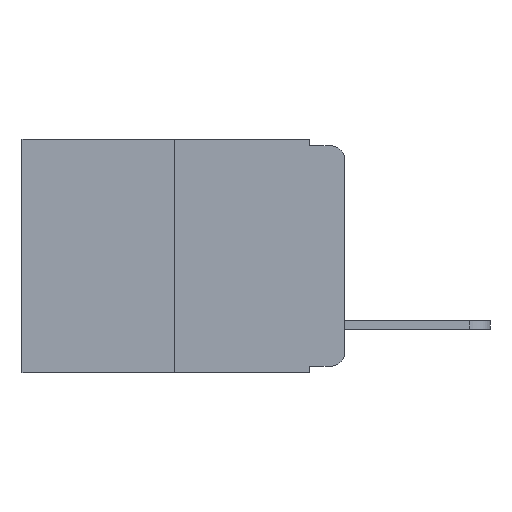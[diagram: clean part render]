
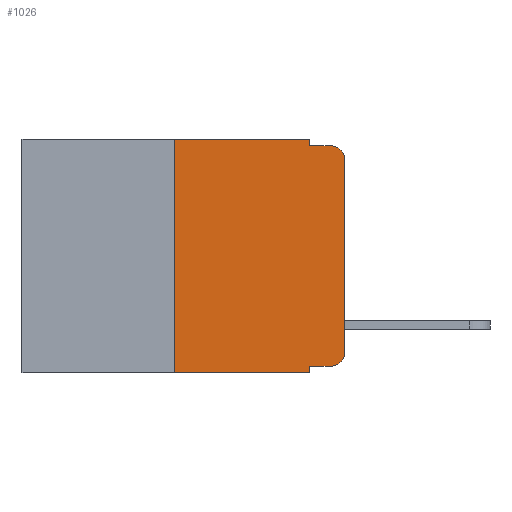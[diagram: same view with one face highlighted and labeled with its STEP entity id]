
A CAD part, left-side view. The second image highlights one B-rep face of the part: STEP entity #1026.
In plain terms, the highlighted planar face has unit normal (-1, 0, 0).
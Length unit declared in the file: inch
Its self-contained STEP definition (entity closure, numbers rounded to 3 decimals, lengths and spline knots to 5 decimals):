
#361 = AXIS2_PLACEMENT_3D ( 'NONE', #1355, #6761, #18345 ) ;
#426 = LINE ( 'NONE', #5913, #13586 ) ;
#1025 = ORIENTED_EDGE ( 'NONE', *, *, #10600, .T. ) ;
#1026 = ADVANCED_FACE ( 'NONE', ( #16637 ), #10312, .F. ) ;
#1355 = CARTESIAN_POINT ( 'NONE',  ( 0., 0.02, -0.03 ) ) ;
#1369 = CARTESIAN_POINT ( 'NONE',  ( 0., 0., 0. ) ) ;
#2298 = VECTOR ( 'NONE', #7303, 39.37008 ) ;
#2314 = CARTESIAN_POINT ( 'NONE',  ( 0., 0.051, 0. ) ) ;
#2365 = VERTEX_POINT ( 'NONE', #13059 ) ;
#3012 = ORIENTED_EDGE ( 'NONE', *, *, #4837, .T. ) ;
#3035 = LINE ( 'NONE', #8787, #15305 ) ;
#4790 = DIRECTION ( 'NONE',  ( 0., 0., -1. ) ) ;
#4837 = EDGE_CURVE ( 'NONE', #14351, #13334, #17825, .T. ) ;
#5016 = EDGE_CURVE ( 'NONE', #2365, #6572, #15844, .T. ) ;
#5109 = EDGE_LOOP ( 'NONE', ( #12586, #6023, #8458, #9532, #16990, #7857, #3012, #16229, #6933, #1025 ) ) ;
#5203 = VECTOR ( 'NONE', #17591, 39.37008 ) ;
#5406 = VERTEX_POINT ( 'NONE', #16628 ) ;
#5456 = CARTESIAN_POINT ( 'NONE',  ( 0., 0.02, -0.333 ) ) ;
#5725 = EDGE_CURVE ( 'NONE', #9122, #7414, #3035, .T. ) ;
#5913 = CARTESIAN_POINT ( 'NONE',  ( 0., 0.473, 0. ) ) ;
#6023 = ORIENTED_EDGE ( 'NONE', *, *, #6155, .T. ) ;
#6078 = DIRECTION ( 'NONE',  ( 1., 0., 0. ) ) ;
#6149 = DIRECTION ( 'NONE',  ( 0., -1., 0. ) ) ;
#6155 = EDGE_CURVE ( 'NONE', #5406, #13989, #14632, .T. ) ;
#6528 = CARTESIAN_POINT ( 'NONE',  ( 0., 0.473, -0.343 ) ) ;
#6572 = VERTEX_POINT ( 'NONE', #5456 ) ;
#6761 = DIRECTION ( 'NONE',  ( -1., 0., 0. ) ) ;
#6933 = ORIENTED_EDGE ( 'NONE', *, *, #5016, .T. ) ;
#7303 = DIRECTION ( 'NONE',  ( 0., 0., 1. ) ) ;
#7414 = VERTEX_POINT ( 'NONE', #11661 ) ;
#7448 = EDGE_CURVE ( 'NONE', #14351, #18371, #14358, .T. ) ;
#7857 = ORIENTED_EDGE ( 'NONE', *, *, #7448, .F. ) ;
#8193 = DIRECTION ( 'NONE',  ( 0., -1., 0. ) ) ;
#8458 = ORIENTED_EDGE ( 'NONE', *, *, #14794, .F. ) ;
#8787 = CARTESIAN_POINT ( 'NONE',  ( 0., 0.051, 0. ) ) ;
#9121 = AXIS2_PLACEMENT_3D ( 'NONE', #17445, #13130, #4790 ) ;
#9122 = VERTEX_POINT ( 'NONE', #2314 ) ;
#9532 = ORIENTED_EDGE ( 'NONE', *, *, #5725, .F. ) ;
#9575 = VECTOR ( 'NONE', #9656, 39.37008 ) ;
#9656 = DIRECTION ( 'NONE',  ( 0., -1., 0. ) ) ;
#9717 = CARTESIAN_POINT ( 'NONE',  ( 0., 0.25, -0.343 ) ) ;
#9768 = DIRECTION ( 'NONE',  ( 0., 0., 1. ) ) ;
#9975 = CARTESIAN_POINT ( 'NONE',  ( 0., 0.25, 0. ) ) ;
#10084 = CARTESIAN_POINT ( 'NONE',  ( 0., 0.25, 0. ) ) ;
#10249 = DIRECTION ( 'NONE',  ( 0., 0., -1. ) ) ;
#10312 = PLANE ( 'NONE',  #12602 ) ;
#10548 = CARTESIAN_POINT ( 'NONE',  ( 0., 0.051, -0.01 ) ) ;
#10600 = EDGE_CURVE ( 'NONE', #6572, #13340, #13796, .T. ) ;
#11089 = CARTESIAN_POINT ( 'NONE',  ( 0., 0.051, -0.333 ) ) ;
#11458 = EDGE_CURVE ( 'NONE', #13340, #5406, #17312, .T. ) ;
#11661 = CARTESIAN_POINT ( 'NONE',  ( 0., 0.051, -0.01 ) ) ;
#11980 = VECTOR ( 'NONE', #9768, 39.37008 ) ;
#12153 = CARTESIAN_POINT ( 'NONE',  ( 0., 0.051, -0.343 ) ) ;
#12586 = ORIENTED_EDGE ( 'NONE', *, *, #11458, .T. ) ;
#12602 = AXIS2_PLACEMENT_3D ( 'NONE', #15947, #6078, #16129 ) ;
#13059 = CARTESIAN_POINT ( 'NONE',  ( 0., 0.051, -0.333 ) ) ;
#13130 = DIRECTION ( 'NONE',  ( -1., 0., 0. ) ) ;
#13334 = VERTEX_POINT ( 'NONE', #12153 ) ;
#13340 = VERTEX_POINT ( 'NONE', #15016 ) ;
#13586 = VECTOR ( 'NONE', #6149, 39.37008 ) ;
#13707 = LINE ( 'NONE', #16288, #5203 ) ;
#13796 = CIRCLE ( 'NONE', #9121, 0.02 ) ;
#13989 = VERTEX_POINT ( 'NONE', #15924 ) ;
#14351 = VERTEX_POINT ( 'NONE', #9717 ) ;
#14358 = LINE ( 'NONE', #10084, #2298 ) ;
#14604 = EDGE_CURVE ( 'NONE', #18371, #9122, #426, .T. ) ;
#14632 = CIRCLE ( 'NONE', #361, 0.02 ) ;
#14794 = EDGE_CURVE ( 'NONE', #7414, #13989, #15841, .T. ) ;
#14828 = DIRECTION ( 'NONE',  ( 0., -1., 0. ) ) ;
#14930 = VECTOR ( 'NONE', #14828, 39.37008 ) ;
#15016 = CARTESIAN_POINT ( 'NONE',  ( 0., 0., -0.313 ) ) ;
#15305 = VECTOR ( 'NONE', #10249, 39.37008 ) ;
#15626 = VECTOR ( 'NONE', #8193, 39.37008 ) ;
#15841 = LINE ( 'NONE', #10548, #14930 ) ;
#15844 = LINE ( 'NONE', #11089, #9575 ) ;
#15924 = CARTESIAN_POINT ( 'NONE',  ( 0., 0.02, -0.01 ) ) ;
#15947 = CARTESIAN_POINT ( 'NONE',  ( 0., 0.473, 0. ) ) ;
#16129 = DIRECTION ( 'NONE',  ( 0., 0., -1. ) ) ;
#16229 = ORIENTED_EDGE ( 'NONE', *, *, #18019, .F. ) ;
#16288 = CARTESIAN_POINT ( 'NONE',  ( 0., 0.051, 0. ) ) ;
#16628 = CARTESIAN_POINT ( 'NONE',  ( 0., 0., -0.03 ) ) ;
#16637 = FACE_OUTER_BOUND ( 'NONE', #5109, .T. ) ;
#16990 = ORIENTED_EDGE ( 'NONE', *, *, #14604, .F. ) ;
#17312 = LINE ( 'NONE', #1369, #11980 ) ;
#17445 = CARTESIAN_POINT ( 'NONE',  ( 0., 0.02, -0.313 ) ) ;
#17591 = DIRECTION ( 'NONE',  ( 0., 0., -1. ) ) ;
#17825 = LINE ( 'NONE', #6528, #15626 ) ;
#18019 = EDGE_CURVE ( 'NONE', #2365, #13334, #13707, .T. ) ;
#18345 = DIRECTION ( 'NONE',  ( 0., 0., -1. ) ) ;
#18371 = VERTEX_POINT ( 'NONE', #9975 ) ;
